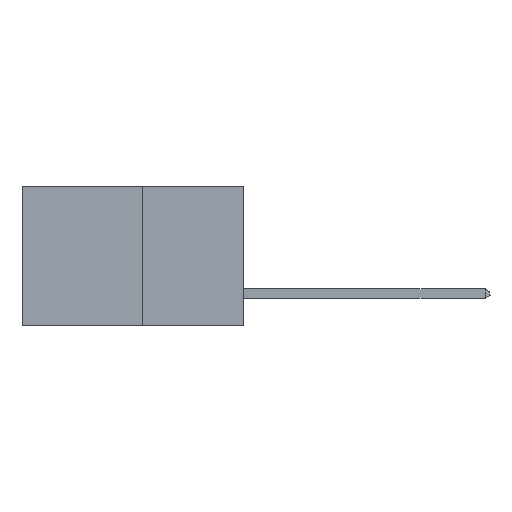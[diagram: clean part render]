
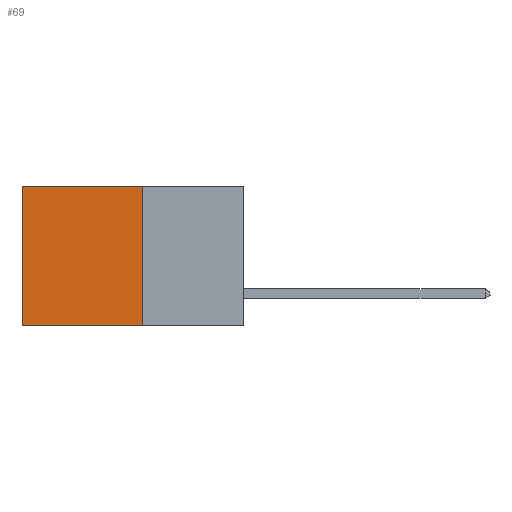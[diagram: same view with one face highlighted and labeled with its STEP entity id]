
A CAD part, left-side view. The second image highlights one B-rep face of the part: STEP entity #69.
In plain terms, the highlighted planar face has unit normal (-1, 0, 0).
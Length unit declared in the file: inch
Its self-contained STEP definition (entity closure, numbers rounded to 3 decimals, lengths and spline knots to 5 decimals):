
#52 = VECTOR ( 'NONE', #4262, 39.37008 ) ;
#69 = ADVANCED_FACE ( 'NONE', ( #3974 ), #11427, .F. ) ;
#434 = EDGE_LOOP ( 'NONE', ( #2061, #1925, #1913, #12642 ) ) ;
#1913 = ORIENTED_EDGE ( 'NONE', *, *, #7970, .F. ) ;
#1925 = ORIENTED_EDGE ( 'NONE', *, *, #13993, .F. ) ;
#2061 = ORIENTED_EDGE ( 'NONE', *, *, #10188, .T. ) ;
#3325 = VERTEX_POINT ( 'NONE', #12788 ) ;
#3772 = LINE ( 'NONE', #4610, #10775 ) ;
#3861 = AXIS2_PLACEMENT_3D ( 'NONE', #6217, #12240, #10648 ) ;
#3938 = VECTOR ( 'NONE', #5801, 39.37008 ) ;
#3974 = FACE_OUTER_BOUND ( 'NONE', #434, .T. ) ;
#4206 = CARTESIAN_POINT ( 'NONE',  ( 0.277, 0.27, 0. ) ) ;
#4262 = DIRECTION ( 'NONE',  ( 0., 1., 0. ) ) ;
#4609 = LINE ( 'NONE', #6859, #10047 ) ;
#4610 = CARTESIAN_POINT ( 'NONE',  ( 0.277, 0.27, -0.37 ) ) ;
#5647 = VERTEX_POINT ( 'NONE', #10362 ) ;
#5800 = DIRECTION ( 'NONE',  ( 0., 1., 0. ) ) ;
#5801 = DIRECTION ( 'NONE',  ( 0., 0., -1. ) ) ;
#5921 = CARTESIAN_POINT ( 'NONE',  ( 0.277, 0.59, -0.37 ) ) ;
#6217 = CARTESIAN_POINT ( 'NONE',  ( 0.277, 0.27, -0.37 ) ) ;
#6260 = LINE ( 'NONE', #4206, #52 ) ;
#6859 = CARTESIAN_POINT ( 'NONE',  ( 0.277, 0.27, -0.37 ) ) ;
#7542 = DIRECTION ( 'NONE',  ( 0., 0., -1. ) ) ;
#7970 = EDGE_CURVE ( 'NONE', #11211, #3325, #4609, .T. ) ;
#8055 = EDGE_CURVE ( 'NONE', #11211, #5647, #6260, .T. ) ;
#10047 = VECTOR ( 'NONE', #7542, 39.37008 ) ;
#10188 = EDGE_CURVE ( 'NONE', #5647, #12747, #13112, .T. ) ;
#10362 = CARTESIAN_POINT ( 'NONE',  ( 0.277, 0.59, 0. ) ) ;
#10648 = DIRECTION ( 'NONE',  ( 0., 0., -1. ) ) ;
#10775 = VECTOR ( 'NONE', #5800, 39.37008 ) ;
#11211 = VERTEX_POINT ( 'NONE', #12302 ) ;
#11427 = PLANE ( 'NONE',  #3861 ) ;
#12240 = DIRECTION ( 'NONE',  ( 1., 0., 0. ) ) ;
#12302 = CARTESIAN_POINT ( 'NONE',  ( 0.277, 0.27, 0. ) ) ;
#12642 = ORIENTED_EDGE ( 'NONE', *, *, #8055, .T. ) ;
#12747 = VERTEX_POINT ( 'NONE', #12787 ) ;
#12787 = CARTESIAN_POINT ( 'NONE',  ( 0.277, 0.59, -0.37 ) ) ;
#12788 = CARTESIAN_POINT ( 'NONE',  ( 0.277, 0.27, -0.37 ) ) ;
#13112 = LINE ( 'NONE', #5921, #3938 ) ;
#13993 = EDGE_CURVE ( 'NONE', #3325, #12747, #3772, .T. ) ;
